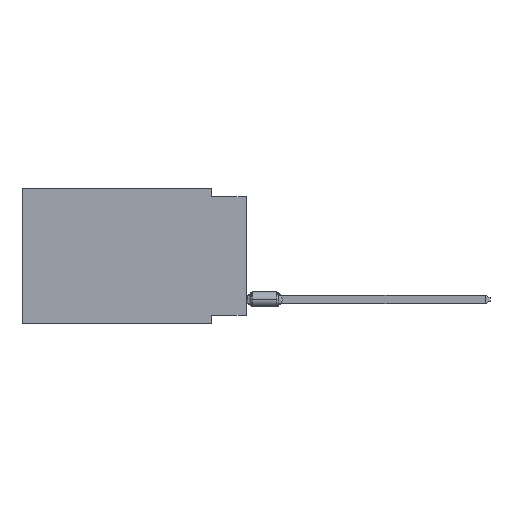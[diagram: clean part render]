
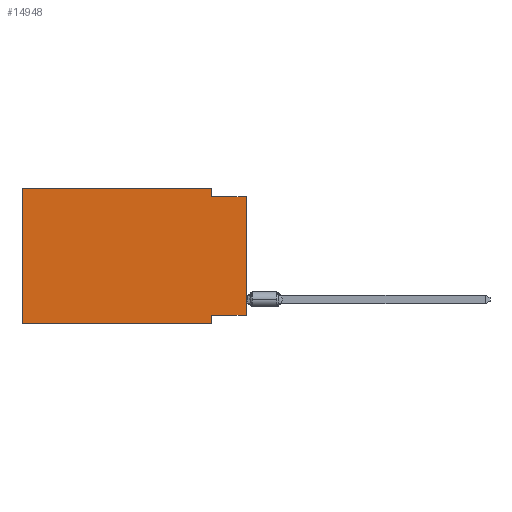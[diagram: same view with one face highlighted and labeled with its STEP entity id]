
A CAD part, left-side view. The second image highlights one B-rep face of the part: STEP entity #14948.
In plain terms, the highlighted planar face has unit normal (-1, 0, 0).
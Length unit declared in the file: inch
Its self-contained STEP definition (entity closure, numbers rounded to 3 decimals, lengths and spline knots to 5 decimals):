
#1332 = VERTEX_POINT ( 'NONE', #18407 ) ;
#1659 = CARTESIAN_POINT ( 'NONE',  ( 0., 0.1, 0. ) ) ;
#2454 = LINE ( 'NONE', #22756, #3143 ) ;
#2910 = ORIENTED_EDGE ( 'NONE', *, *, #6924, .T. ) ;
#3143 = VECTOR ( 'NONE', #5815, 39.37008 ) ;
#3432 = VERTEX_POINT ( 'NONE', #10918 ) ;
#3913 = ORIENTED_EDGE ( 'NONE', *, *, #8014, .F. ) ;
#4493 = CARTESIAN_POINT ( 'NONE',  ( 0., 0.645, 0. ) ) ;
#4673 = CARTESIAN_POINT ( 'NONE',  ( 0., 0.1, 0. ) ) ;
#5652 = LINE ( 'NONE', #13116, #20442 ) ;
#5815 = DIRECTION ( 'NONE',  ( 0., -1., 0. ) ) ;
#6045 = AXIS2_PLACEMENT_3D ( 'NONE', #4493, #18935, #8091 ) ;
#6169 = PLANE ( 'NONE',  #6045 ) ;
#6200 = DIRECTION ( 'NONE',  ( 0., 0., -1. ) ) ;
#6256 = VECTOR ( 'NONE', #21804, 39.37008 ) ;
#6924 = EDGE_CURVE ( 'NONE', #17816, #1332, #10010, .T. ) ;
#7127 = VERTEX_POINT ( 'NONE', #12868 ) ;
#7475 = EDGE_LOOP ( 'NONE', ( #11347, #8267, #16457, #3913, #21425, #2910, #12519, #13214 ) ) ;
#8014 = EDGE_CURVE ( 'NONE', #7127, #21471, #2454, .T. ) ;
#8091 = DIRECTION ( 'NONE',  ( 0., 0., -1. ) ) ;
#8267 = ORIENTED_EDGE ( 'NONE', *, *, #22192, .F. ) ;
#8755 = LINE ( 'NONE', #1659, #19665 ) ;
#8969 = LINE ( 'NONE', #16413, #6256 ) ;
#10010 = LINE ( 'NONE', #11950, #11554 ) ;
#10282 = EDGE_CURVE ( 'NONE', #21471, #12873, #8755, .T. ) ;
#10302 = LINE ( 'NONE', #23376, #15131 ) ;
#10375 = DIRECTION ( 'NONE',  ( 0., -1., 0. ) ) ;
#10918 = CARTESIAN_POINT ( 'NONE',  ( 0., 0., -0.025 ) ) ;
#11145 = CARTESIAN_POINT ( 'NONE',  ( 0., 0., -0.025 ) ) ;
#11190 = EDGE_CURVE ( 'NONE', #12398, #3432, #5652, .T. ) ;
#11347 = ORIENTED_EDGE ( 'NONE', *, *, #11190, .T. ) ;
#11554 = VECTOR ( 'NONE', #10375, 39.37008 ) ;
#11950 = CARTESIAN_POINT ( 'NONE',  ( 0., 0.645, -0.39 ) ) ;
#12398 = VERTEX_POINT ( 'NONE', #20305 ) ;
#12519 = ORIENTED_EDGE ( 'NONE', *, *, #22297, .F. ) ;
#12868 = CARTESIAN_POINT ( 'NONE',  ( 0., 0.645, 0. ) ) ;
#12873 = VERTEX_POINT ( 'NONE', #20055 ) ;
#13075 = LINE ( 'NONE', #11145, #19357 ) ;
#13116 = CARTESIAN_POINT ( 'NONE',  ( 0., 0., 0. ) ) ;
#13214 = ORIENTED_EDGE ( 'NONE', *, *, #21585, .F. ) ;
#13791 = DIRECTION ( 'NONE',  ( 0., 0., 1. ) ) ;
#14948 = ADVANCED_FACE ( 'NONE', ( #22626 ), #6169, .F. ) ;
#15131 = VECTOR ( 'NONE', #13791, 39.37008 ) ;
#16354 = CARTESIAN_POINT ( 'NONE',  ( 0., 0.1, -0.365 ) ) ;
#16413 = CARTESIAN_POINT ( 'NONE',  ( 0., 0., -0.365 ) ) ;
#16457 = ORIENTED_EDGE ( 'NONE', *, *, #10282, .F. ) ;
#16864 = VERTEX_POINT ( 'NONE', #16354 ) ;
#17478 = CARTESIAN_POINT ( 'NONE',  ( 0., 0.645, -0.39 ) ) ;
#17816 = VERTEX_POINT ( 'NONE', #17478 ) ;
#18374 = DIRECTION ( 'NONE',  ( 0., -1., 0. ) ) ;
#18407 = CARTESIAN_POINT ( 'NONE',  ( 0., 0.1, -0.39 ) ) ;
#18935 = DIRECTION ( 'NONE',  ( 1., 0., 0. ) ) ;
#18969 = CARTESIAN_POINT ( 'NONE',  ( 0., 0.1, -0.39 ) ) ;
#19357 = VECTOR ( 'NONE', #18374, 39.37008 ) ;
#19665 = VECTOR ( 'NONE', #19923, 39.37008 ) ;
#19923 = DIRECTION ( 'NONE',  ( 0., 0., -1. ) ) ;
#20055 = CARTESIAN_POINT ( 'NONE',  ( 0., 0.1, -0.025 ) ) ;
#20305 = CARTESIAN_POINT ( 'NONE',  ( 0., 0., -0.365 ) ) ;
#20442 = VECTOR ( 'NONE', #21866, 39.37008 ) ;
#21425 = ORIENTED_EDGE ( 'NONE', *, *, #23716, .F. ) ;
#21471 = VERTEX_POINT ( 'NONE', #4673 ) ;
#21585 = EDGE_CURVE ( 'NONE', #12398, #16864, #8969, .T. ) ;
#21804 = DIRECTION ( 'NONE',  ( 0., 1., 0. ) ) ;
#21866 = DIRECTION ( 'NONE',  ( 0., 0., 1. ) ) ;
#22192 = EDGE_CURVE ( 'NONE', #12873, #3432, #13075, .T. ) ;
#22297 = EDGE_CURVE ( 'NONE', #16864, #1332, #22662, .T. ) ;
#22420 = VECTOR ( 'NONE', #6200, 39.37008 ) ;
#22626 = FACE_OUTER_BOUND ( 'NONE', #7475, .T. ) ;
#22662 = LINE ( 'NONE', #18969, #22420 ) ;
#22756 = CARTESIAN_POINT ( 'NONE',  ( 0., 0.645, 0. ) ) ;
#23376 = CARTESIAN_POINT ( 'NONE',  ( 0., 0.645, 0. ) ) ;
#23716 = EDGE_CURVE ( 'NONE', #17816, #7127, #10302, .T. ) ;
